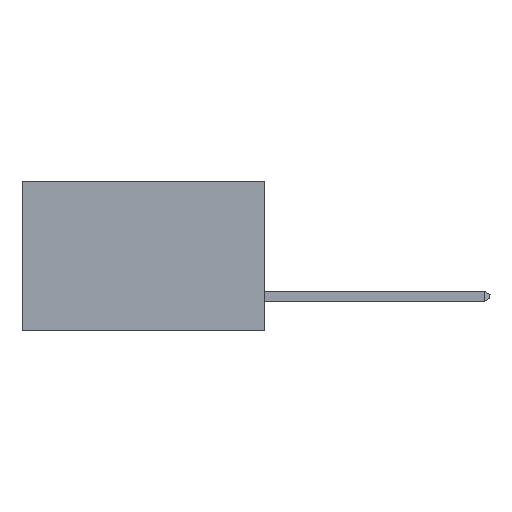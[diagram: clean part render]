
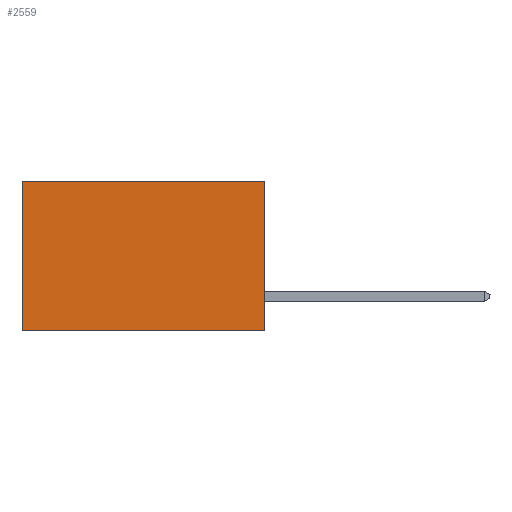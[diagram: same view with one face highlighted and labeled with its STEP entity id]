
A CAD part, left-side view. The second image highlights one B-rep face of the part: STEP entity #2559.
In plain terms, the highlighted planar face has unit normal (-1, 0, 0).
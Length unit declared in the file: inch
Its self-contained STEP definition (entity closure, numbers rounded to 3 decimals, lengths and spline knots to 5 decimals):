
#461 = FACE_OUTER_BOUND ( 'NONE', #10915, .T. ) ;
#2559 = ADVANCED_FACE ( 'NONE', ( #461 ), #10105, .F. ) ;
#2925 = VERTEX_POINT ( 'NONE', #31342 ) ;
#3265 = VERTEX_POINT ( 'NONE', #15739 ) ;
#3559 = VECTOR ( 'NONE', #24863, 39.37008 ) ;
#5740 = CARTESIAN_POINT ( 'NONE',  ( 0.298, 0., 0. ) ) ;
#5830 = LINE ( 'NONE', #10020, #3559 ) ;
#7191 = CARTESIAN_POINT ( 'NONE',  ( 0.298, 0., -0.37 ) ) ;
#7625 = AXIS2_PLACEMENT_3D ( 'NONE', #24726, #10303, #15011 ) ;
#7631 = VERTEX_POINT ( 'NONE', #8241 ) ;
#8241 = CARTESIAN_POINT ( 'NONE',  ( 0.298, 0.6, -0.37 ) ) ;
#8870 = VERTEX_POINT ( 'NONE', #8897 ) ;
#8897 = CARTESIAN_POINT ( 'NONE',  ( 0.298, 0.6, 0. ) ) ;
#9058 = DIRECTION ( 'NONE',  ( 0., 0., -1. ) ) ;
#9746 = VECTOR ( 'NONE', #10667, 39.37008 ) ;
#10020 = CARTESIAN_POINT ( 'NONE',  ( 0.298, 0.6, 0. ) ) ;
#10105 = PLANE ( 'NONE',  #7625 ) ;
#10303 = DIRECTION ( 'NONE',  ( 1., 0., 0. ) ) ;
#10667 = DIRECTION ( 'NONE',  ( 0., 1., 0. ) ) ;
#10915 = EDGE_LOOP ( 'NONE', ( #20760, #12768, #22214, #22883 ) ) ;
#12768 = ORIENTED_EDGE ( 'NONE', *, *, #22335, .F. ) ;
#13016 = VECTOR ( 'NONE', #24234, 39.37008 ) ;
#13062 = VECTOR ( 'NONE', #9058, 39.37008 ) ;
#14706 = LINE ( 'NONE', #5740, #9746 ) ;
#15011 = DIRECTION ( 'NONE',  ( 0., 0., -1. ) ) ;
#15739 = CARTESIAN_POINT ( 'NONE',  ( 0.298, 0., -0.37 ) ) ;
#16489 = EDGE_CURVE ( 'NONE', #2925, #3265, #22979, .T. ) ;
#16639 = CARTESIAN_POINT ( 'NONE',  ( 0.298, 0., 0. ) ) ;
#19503 = LINE ( 'NONE', #7191, #13016 ) ;
#20088 = EDGE_CURVE ( 'NONE', #2925, #8870, #14706, .T. ) ;
#20760 = ORIENTED_EDGE ( 'NONE', *, *, #28422, .T. ) ;
#22214 = ORIENTED_EDGE ( 'NONE', *, *, #16489, .F. ) ;
#22335 = EDGE_CURVE ( 'NONE', #3265, #7631, #19503, .T. ) ;
#22883 = ORIENTED_EDGE ( 'NONE', *, *, #20088, .T. ) ;
#22979 = LINE ( 'NONE', #16639, #13062 ) ;
#24234 = DIRECTION ( 'NONE',  ( 0., 1., 0. ) ) ;
#24726 = CARTESIAN_POINT ( 'NONE',  ( 0.298, 0., 0. ) ) ;
#24863 = DIRECTION ( 'NONE',  ( 0., 0., -1. ) ) ;
#28422 = EDGE_CURVE ( 'NONE', #8870, #7631, #5830, .T. ) ;
#31342 = CARTESIAN_POINT ( 'NONE',  ( 0.298, 0., 0. ) ) ;
